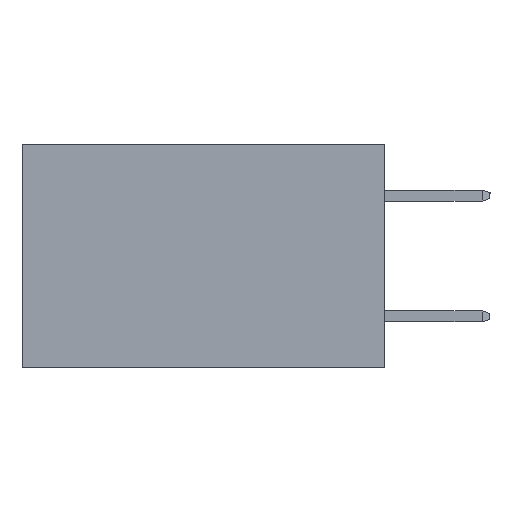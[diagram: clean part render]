
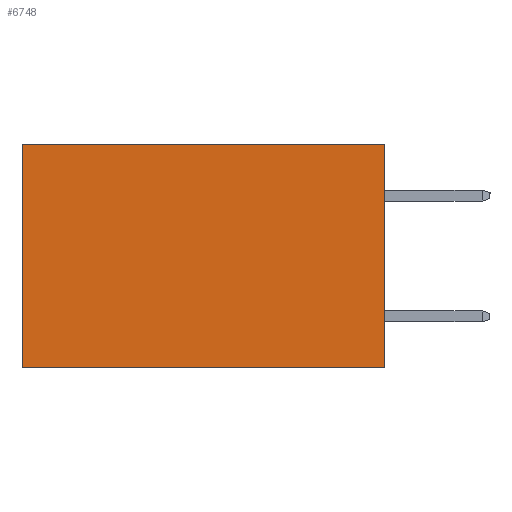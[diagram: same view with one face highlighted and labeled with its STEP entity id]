
A CAD part, left-side view. The second image highlights one B-rep face of the part: STEP entity #6748.
In plain terms, the highlighted planar face has unit normal (-1, 0, 0).
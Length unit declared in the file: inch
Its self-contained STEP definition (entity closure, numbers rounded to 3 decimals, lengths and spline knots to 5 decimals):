
#31 = ORIENTED_EDGE ( 'NONE', *, *, #15015, .F. ) ;
#93 = VECTOR ( 'NONE', #8295, 39.37008 ) ;
#2699 = VERTEX_POINT ( 'NONE', #6403 ) ;
#3090 = CARTESIAN_POINT ( 'NONE',  ( 0.2615, 0., -0.37 ) ) ;
#3109 = CARTESIAN_POINT ( 'NONE',  ( 0.2615, 0., 0. ) ) ;
#4266 = LINE ( 'NONE', #7643, #14971 ) ;
#5034 = EDGE_CURVE ( 'NONE', #2699, #5926, #21685, .T. ) ;
#5909 = CARTESIAN_POINT ( 'NONE',  ( 0.2615, 0., -0.37 ) ) ;
#5926 = VERTEX_POINT ( 'NONE', #9990 ) ;
#6308 = VECTOR ( 'NONE', #15134, 39.37008 ) ;
#6403 = CARTESIAN_POINT ( 'NONE',  ( 0.2615, 0.6, 0. ) ) ;
#6748 = ADVANCED_FACE ( 'NONE', ( #17208 ), #13950, .F. ) ;
#7021 = VERTEX_POINT ( 'NONE', #14831 ) ;
#7471 = EDGE_CURVE ( 'NONE', #7021, #2699, #18535, .T. ) ;
#7643 = CARTESIAN_POINT ( 'NONE',  ( 0.2615, 0., -0.37 ) ) ;
#8295 = DIRECTION ( 'NONE',  ( 0., 0., -1. ) ) ;
#9987 = DIRECTION ( 'NONE',  ( 0., 1., 0. ) ) ;
#9990 = CARTESIAN_POINT ( 'NONE',  ( 0.2615, 0.6, -0.37 ) ) ;
#10292 = LINE ( 'NONE', #3090, #6308 ) ;
#10982 = ORIENTED_EDGE ( 'NONE', *, *, #7471, .T. ) ;
#11220 = VERTEX_POINT ( 'NONE', #5909 ) ;
#13800 = EDGE_CURVE ( 'NONE', #7021, #11220, #10292, .T. ) ;
#13823 = DIRECTION ( 'NONE',  ( 0., 0., -1. ) ) ;
#13950 = PLANE ( 'NONE',  #17015 ) ;
#14831 = CARTESIAN_POINT ( 'NONE',  ( 0.2615, 0., 0. ) ) ;
#14971 = VECTOR ( 'NONE', #19687, 39.37008 ) ;
#15015 = EDGE_CURVE ( 'NONE', #11220, #5926, #4266, .T. ) ;
#15134 = DIRECTION ( 'NONE',  ( 0., 0., -1. ) ) ;
#15617 = CARTESIAN_POINT ( 'NONE',  ( 0.2615, 0., -0.37 ) ) ;
#17015 = AXIS2_PLACEMENT_3D ( 'NONE', #15617, #18769, #13823 ) ;
#17208 = FACE_OUTER_BOUND ( 'NONE', #17689, .T. ) ;
#17689 = EDGE_LOOP ( 'NONE', ( #18775, #31, #18406, #10982 ) ) ;
#17777 = VECTOR ( 'NONE', #9987, 39.37008 ) ;
#18406 = ORIENTED_EDGE ( 'NONE', *, *, #13800, .F. ) ;
#18535 = LINE ( 'NONE', #3109, #17777 ) ;
#18769 = DIRECTION ( 'NONE',  ( 1., 0., 0. ) ) ;
#18775 = ORIENTED_EDGE ( 'NONE', *, *, #5034, .T. ) ;
#19687 = DIRECTION ( 'NONE',  ( 0., 1., 0. ) ) ;
#20013 = CARTESIAN_POINT ( 'NONE',  ( 0.2615, 0.6, -0.37 ) ) ;
#21685 = LINE ( 'NONE', #20013, #93 ) ;
